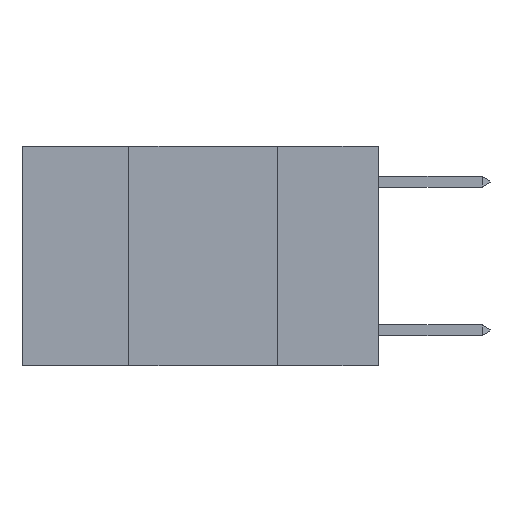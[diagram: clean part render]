
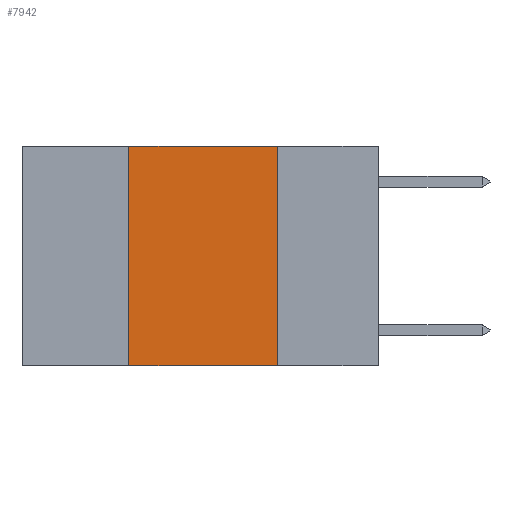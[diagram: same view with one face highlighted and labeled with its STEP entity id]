
A CAD part, left-side view. The second image highlights one B-rep face of the part: STEP entity #7942.
In plain terms, the highlighted planar face has unit normal (-1, 0, 0).
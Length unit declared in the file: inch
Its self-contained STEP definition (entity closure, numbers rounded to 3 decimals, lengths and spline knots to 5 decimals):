
#475 = DIRECTION ( 'NONE',  ( 0., 0., 1. ) ) ;
#681 = LINE ( 'NONE', #13006, #13992 ) ;
#1423 = EDGE_CURVE ( 'NONE', #8171, #10052, #681, .T. ) ;
#1660 = DIRECTION ( 'NONE',  ( 0., -1., 0. ) ) ;
#2254 = CARTESIAN_POINT ( 'NONE',  ( 0., 0.42, -0.37 ) ) ;
#2652 = EDGE_CURVE ( 'NONE', #3055, #11388, #4046, .T. ) ;
#2847 = DIRECTION ( 'NONE',  ( 0., -1., 0. ) ) ;
#3055 = VERTEX_POINT ( 'NONE', #2254 ) ;
#3516 = CARTESIAN_POINT ( 'NONE',  ( 0., 0.42, 0. ) ) ;
#4046 = LINE ( 'NONE', #8516, #8848 ) ;
#5118 = VECTOR ( 'NONE', #13516, 39.37008 ) ;
#5279 = ORIENTED_EDGE ( 'NONE', *, *, #2652, .T. ) ;
#5562 = LINE ( 'NONE', #12326, #5118 ) ;
#6066 = VECTOR ( 'NONE', #475, 39.37008 ) ;
#6096 = PLANE ( 'NONE',  #9380 ) ;
#6144 = CARTESIAN_POINT ( 'NONE',  ( 0., 0.17, 0. ) ) ;
#6167 = CARTESIAN_POINT ( 'NONE',  ( 0., 0.17, -0.37 ) ) ;
#6418 = CARTESIAN_POINT ( 'NONE',  ( 0., 0.42, 0. ) ) ;
#7376 = LINE ( 'NONE', #6418, #6066 ) ;
#7942 = ADVANCED_FACE ( 'NONE', ( #10495 ), #6096, .F. ) ;
#8171 = VERTEX_POINT ( 'NONE', #3516 ) ;
#8516 = CARTESIAN_POINT ( 'NONE',  ( 0., 0.6, -0.37 ) ) ;
#8629 = EDGE_CURVE ( 'NONE', #10052, #11388, #5562, .T. ) ;
#8848 = VECTOR ( 'NONE', #1660, 39.37008 ) ;
#9125 = EDGE_LOOP ( 'NONE', ( #11250, #12863, #13176, #5279 ) ) ;
#9219 = EDGE_CURVE ( 'NONE', #3055, #8171, #7376, .T. ) ;
#9256 = DIRECTION ( 'NONE',  ( 0., 0., -1. ) ) ;
#9380 = AXIS2_PLACEMENT_3D ( 'NONE', #10362, #9388, #9256 ) ;
#9388 = DIRECTION ( 'NONE',  ( 1., 0., 0. ) ) ;
#10052 = VERTEX_POINT ( 'NONE', #6144 ) ;
#10362 = CARTESIAN_POINT ( 'NONE',  ( 0., 0.6, 0. ) ) ;
#10495 = FACE_OUTER_BOUND ( 'NONE', #9125, .T. ) ;
#11250 = ORIENTED_EDGE ( 'NONE', *, *, #8629, .F. ) ;
#11388 = VERTEX_POINT ( 'NONE', #6167 ) ;
#12326 = CARTESIAN_POINT ( 'NONE',  ( 0., 0.17, 0. ) ) ;
#12863 = ORIENTED_EDGE ( 'NONE', *, *, #1423, .F. ) ;
#13006 = CARTESIAN_POINT ( 'NONE',  ( 0., 0.6, 0. ) ) ;
#13176 = ORIENTED_EDGE ( 'NONE', *, *, #9219, .F. ) ;
#13516 = DIRECTION ( 'NONE',  ( 0., 0., -1. ) ) ;
#13992 = VECTOR ( 'NONE', #2847, 39.37008 ) ;
